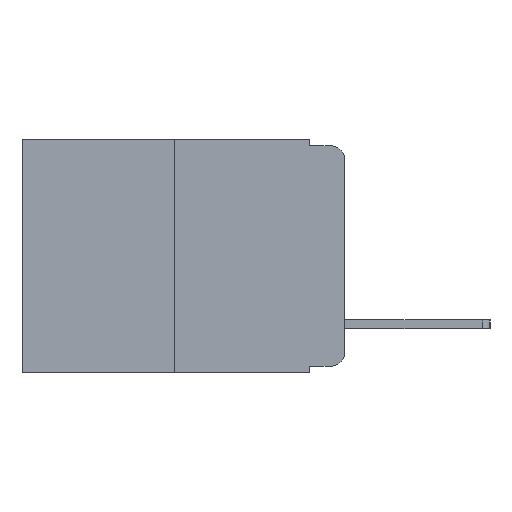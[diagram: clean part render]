
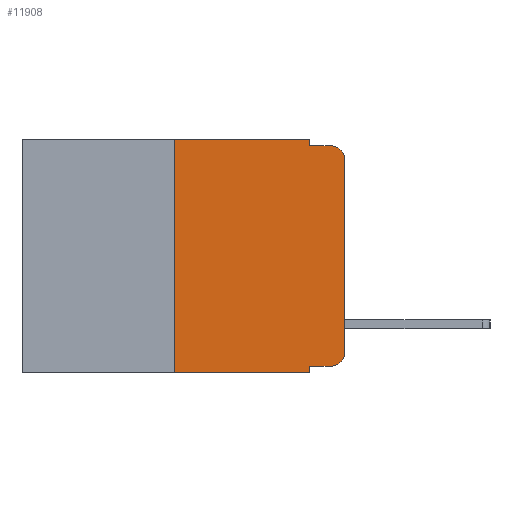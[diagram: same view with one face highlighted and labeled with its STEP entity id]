
A CAD part, left-side view. The second image highlights one B-rep face of the part: STEP entity #11908.
In plain terms, the highlighted planar face has unit normal (-1, 0, 0).
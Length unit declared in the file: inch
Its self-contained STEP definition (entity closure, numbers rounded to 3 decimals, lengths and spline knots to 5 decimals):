
#28 = CARTESIAN_POINT ( 'NONE',  ( 0., 0., -0.03 ) ) ;
#562 = ORIENTED_EDGE ( 'NONE', *, *, #11661, .F. ) ;
#615 = LINE ( 'NONE', #9415, #16250 ) ;
#718 = CARTESIAN_POINT ( 'NONE',  ( 0., 0.473, 0. ) ) ;
#1680 = ORIENTED_EDGE ( 'NONE', *, *, #8654, .F. ) ;
#2191 = CARTESIAN_POINT ( 'NONE',  ( 0., 0.051, 0. ) ) ;
#2220 = EDGE_CURVE ( 'NONE', #5419, #16670, #3526, .T. ) ;
#2392 = EDGE_CURVE ( 'NONE', #15478, #17169, #18901, .T. ) ;
#2527 = DIRECTION ( 'NONE',  ( 0., 0., -1. ) ) ;
#2583 = CARTESIAN_POINT ( 'NONE',  ( 0., 0.051, -0.333 ) ) ;
#2645 = CARTESIAN_POINT ( 'NONE',  ( 0., 0.051, -0.01 ) ) ;
#2945 = EDGE_CURVE ( 'NONE', #14907, #19411, #3507, .T. ) ;
#3203 = LINE ( 'NONE', #5938, #14478 ) ;
#3395 = EDGE_CURVE ( 'NONE', #5419, #19411, #3203, .T. ) ;
#3404 = DIRECTION ( 'NONE',  ( -1., 0., 0. ) ) ;
#3478 = DIRECTION ( 'NONE',  ( 0., 0., 1. ) ) ;
#3507 = LINE ( 'NONE', #14474, #7214 ) ;
#3526 = LINE ( 'NONE', #2583, #8186 ) ;
#3679 = VERTEX_POINT ( 'NONE', #2191 ) ;
#3774 = EDGE_CURVE ( 'NONE', #17095, #3679, #16990, .T. ) ;
#4170 = CARTESIAN_POINT ( 'NONE',  ( 0., 0.051, -0.333 ) ) ;
#5024 = CARTESIAN_POINT ( 'NONE',  ( 0., 0.25, 0. ) ) ;
#5419 = VERTEX_POINT ( 'NONE', #4170 ) ;
#5604 = ORIENTED_EDGE ( 'NONE', *, *, #12651, .F. ) ;
#5607 = CARTESIAN_POINT ( 'NONE',  ( 0., 0.25, 0. ) ) ;
#5938 = CARTESIAN_POINT ( 'NONE',  ( 0., 0.051, 0. ) ) ;
#6087 = ORIENTED_EDGE ( 'NONE', *, *, #2945, .T. ) ;
#6101 = DIRECTION ( 'NONE',  ( -1., 0., 0. ) ) ;
#7067 = ORIENTED_EDGE ( 'NONE', *, *, #2220, .T. ) ;
#7214 = VECTOR ( 'NONE', #14542, 39.37008 ) ;
#7308 = PLANE ( 'NONE',  #15846 ) ;
#8186 = VECTOR ( 'NONE', #11900, 39.37008 ) ;
#8522 = CARTESIAN_POINT ( 'NONE',  ( 0., 0.051, -0.343 ) ) ;
#8654 = EDGE_CURVE ( 'NONE', #14907, #17095, #14245, .T. ) ;
#8744 = ORIENTED_EDGE ( 'NONE', *, *, #12175, .T. ) ;
#8784 = VERTEX_POINT ( 'NONE', #18891 ) ;
#8805 = LINE ( 'NONE', #16610, #12300 ) ;
#9020 = FACE_OUTER_BOUND ( 'NONE', #12019, .T. ) ;
#9022 = VERTEX_POINT ( 'NONE', #2645 ) ;
#9064 = VECTOR ( 'NONE', #16324, 39.37008 ) ;
#9182 = CARTESIAN_POINT ( 'NONE',  ( 0., 0.02, -0.333 ) ) ;
#9238 = LINE ( 'NONE', #12547, #17152 ) ;
#9415 = CARTESIAN_POINT ( 'NONE',  ( 0., 0., 0. ) ) ;
#10301 = VECTOR ( 'NONE', #3478, 39.37008 ) ;
#11661 = EDGE_CURVE ( 'NONE', #9022, #17169, #8805, .T. ) ;
#11850 = DIRECTION ( 'NONE',  ( 1., 0., 0. ) ) ;
#11900 = DIRECTION ( 'NONE',  ( 0., -1., 0. ) ) ;
#11908 = ADVANCED_FACE ( 'NONE', ( #9020 ), #7308, .F. ) ;
#12019 = EDGE_LOOP ( 'NONE', ( #8744, #16667, #562, #5604, #17600, #1680, #6087, #18507, #7067, #15515 ) ) ;
#12175 = EDGE_CURVE ( 'NONE', #8784, #15478, #615, .T. ) ;
#12300 = VECTOR ( 'NONE', #18730, 39.37008 ) ;
#12547 = CARTESIAN_POINT ( 'NONE',  ( 0., 0.051, 0. ) ) ;
#12581 = CARTESIAN_POINT ( 'NONE',  ( 0., 0.02, -0.03 ) ) ;
#12651 = EDGE_CURVE ( 'NONE', #3679, #9022, #9238, .T. ) ;
#13588 = AXIS2_PLACEMENT_3D ( 'NONE', #15135, #6101, #16626 ) ;
#14098 = DIRECTION ( 'NONE',  ( 0., 0., -1. ) ) ;
#14245 = LINE ( 'NONE', #5024, #10301 ) ;
#14474 = CARTESIAN_POINT ( 'NONE',  ( 0., 0.473, -0.343 ) ) ;
#14478 = VECTOR ( 'NONE', #17888, 39.37008 ) ;
#14542 = DIRECTION ( 'NONE',  ( 0., -1., 0. ) ) ;
#14790 = CARTESIAN_POINT ( 'NONE',  ( 0., 0.02, -0.01 ) ) ;
#14836 = CARTESIAN_POINT ( 'NONE',  ( 0., 0.473, 0. ) ) ;
#14907 = VERTEX_POINT ( 'NONE', #16013 ) ;
#15135 = CARTESIAN_POINT ( 'NONE',  ( 0., 0.02, -0.313 ) ) ;
#15478 = VERTEX_POINT ( 'NONE', #28 ) ;
#15515 = ORIENTED_EDGE ( 'NONE', *, *, #19005, .T. ) ;
#15846 = AXIS2_PLACEMENT_3D ( 'NONE', #718, #11850, #2527 ) ;
#16013 = CARTESIAN_POINT ( 'NONE',  ( 0., 0.25, -0.343 ) ) ;
#16250 = VECTOR ( 'NONE', #19734, 39.37008 ) ;
#16324 = DIRECTION ( 'NONE',  ( 0., -1., 0. ) ) ;
#16610 = CARTESIAN_POINT ( 'NONE',  ( 0., 0.051, -0.01 ) ) ;
#16626 = DIRECTION ( 'NONE',  ( 0., 0., -1. ) ) ;
#16667 = ORIENTED_EDGE ( 'NONE', *, *, #2392, .T. ) ;
#16670 = VERTEX_POINT ( 'NONE', #9182 ) ;
#16990 = LINE ( 'NONE', #14836, #9064 ) ;
#17095 = VERTEX_POINT ( 'NONE', #5607 ) ;
#17152 = VECTOR ( 'NONE', #18456, 39.37008 ) ;
#17169 = VERTEX_POINT ( 'NONE', #14790 ) ;
#17548 = AXIS2_PLACEMENT_3D ( 'NONE', #12581, #3404, #14098 ) ;
#17600 = ORIENTED_EDGE ( 'NONE', *, *, #3774, .F. ) ;
#17888 = DIRECTION ( 'NONE',  ( 0., 0., -1. ) ) ;
#18456 = DIRECTION ( 'NONE',  ( 0., 0., -1. ) ) ;
#18507 = ORIENTED_EDGE ( 'NONE', *, *, #3395, .F. ) ;
#18730 = DIRECTION ( 'NONE',  ( 0., -1., 0. ) ) ;
#18891 = CARTESIAN_POINT ( 'NONE',  ( 0., 0., -0.313 ) ) ;
#18901 = CIRCLE ( 'NONE', #17548, 0.02 ) ;
#19005 = EDGE_CURVE ( 'NONE', #16670, #8784, #19400, .T. ) ;
#19400 = CIRCLE ( 'NONE', #13588, 0.02 ) ;
#19411 = VERTEX_POINT ( 'NONE', #8522 ) ;
#19734 = DIRECTION ( 'NONE',  ( 0., 0., 1. ) ) ;
